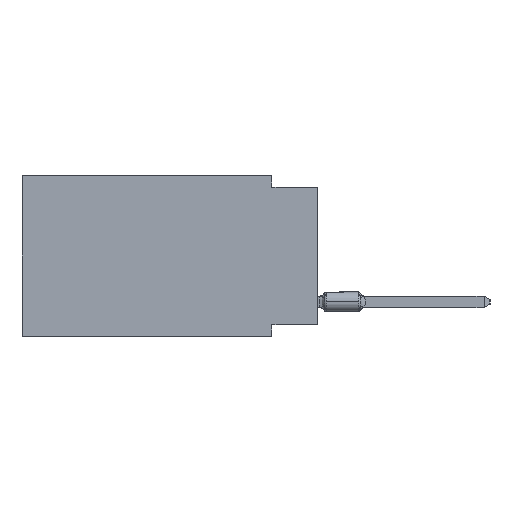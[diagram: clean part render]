
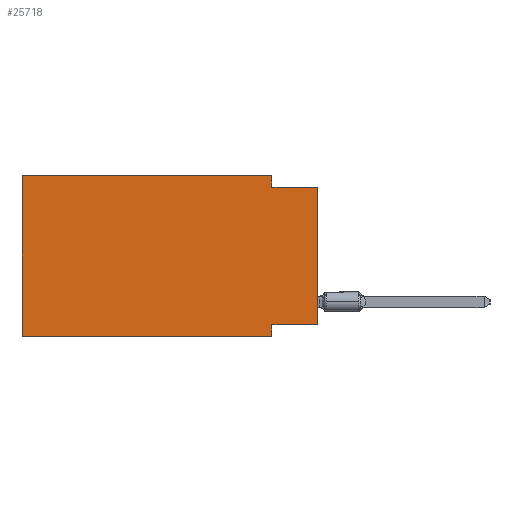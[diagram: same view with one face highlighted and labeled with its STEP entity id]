
A CAD part, left-side view. The second image highlights one B-rep face of the part: STEP entity #25718.
In plain terms, the highlighted planar face has unit normal (-1, 0, 0).
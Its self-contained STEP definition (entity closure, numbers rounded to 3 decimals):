
#2215 = LINE ( 'NONE', #15196, #21872 ) ;
#2265 = DIRECTION ( 'NONE',  ( 0., -1., 0. ) ) ;
#2709 = CARTESIAN_POINT ( 'NONE',  ( 0., 2.54, -8.89 ) ) ;
#3621 = LINE ( 'NONE', #29125, #31498 ) ;
#4980 = CARTESIAN_POINT ( 'NONE',  ( 0., 0., -0.635 ) ) ;
#5808 = EDGE_CURVE ( 'NONE', #7178, #38182, #6358, .T. ) ;
#6358 = LINE ( 'NONE', #35792, #7038 ) ;
#7038 = VECTOR ( 'NONE', #32453, 1000. ) ;
#7178 = VERTEX_POINT ( 'NONE', #31589 ) ;
#7741 = ORIENTED_EDGE ( 'NONE', *, *, #18142, .T. ) ;
#9177 = EDGE_CURVE ( 'NONE', #12048, #35317, #15243, .T. ) ;
#9203 = ORIENTED_EDGE ( 'NONE', *, *, #9177, .F. ) ;
#10192 = CARTESIAN_POINT ( 'NONE',  ( 0., 0., -8.255 ) ) ;
#10745 = DIRECTION ( 'NONE',  ( 0., -1., 0. ) ) ;
#11091 = CARTESIAN_POINT ( 'NONE',  ( 0., 16.383, 0. ) ) ;
#11846 = DIRECTION ( 'NONE',  ( 0., 0., 1. ) ) ;
#12048 = VERTEX_POINT ( 'NONE', #10192 ) ;
#13253 = VECTOR ( 'NONE', #35479, 1000. ) ;
#14845 = VERTEX_POINT ( 'NONE', #4980 ) ;
#15196 = CARTESIAN_POINT ( 'NONE',  ( 0., 0., 0. ) ) ;
#15243 = LINE ( 'NONE', #37995, #39353 ) ;
#15886 = VECTOR ( 'NONE', #40746, 1000. ) ;
#16350 = VERTEX_POINT ( 'NONE', #19687 ) ;
#16980 = PLANE ( 'NONE',  #17020 ) ;
#17020 = AXIS2_PLACEMENT_3D ( 'NONE', #11091, #36781, #39919 ) ;
#17247 = VECTOR ( 'NONE', #2265, 1000. ) ;
#18142 = EDGE_CURVE ( 'NONE', #7178, #28226, #3621, .T. ) ;
#18381 = CARTESIAN_POINT ( 'NONE',  ( 0., 0., -0.635 ) ) ;
#19687 = CARTESIAN_POINT ( 'NONE',  ( 0., 2.54, -0.635 ) ) ;
#19945 = ORIENTED_EDGE ( 'NONE', *, *, #35447, .F. ) ;
#20301 = FACE_OUTER_BOUND ( 'NONE', #33129, .T. ) ;
#20657 = ORIENTED_EDGE ( 'NONE', *, *, #34658, .F. ) ;
#21872 = VECTOR ( 'NONE', #11846, 1000. ) ;
#22324 = DIRECTION ( 'NONE',  ( 0., 1., 0. ) ) ;
#22740 = CARTESIAN_POINT ( 'NONE',  ( 0., 2.54, 0. ) ) ;
#22844 = DIRECTION ( 'NONE',  ( 0., -1., 0. ) ) ;
#25043 = LINE ( 'NONE', #22740, #13253 ) ;
#25348 = EDGE_CURVE ( 'NONE', #38182, #28399, #36027, .T. ) ;
#25436 = ORIENTED_EDGE ( 'NONE', *, *, #5808, .F. ) ;
#25718 = ADVANCED_FACE ( 'NONE', ( #20301 ), #16980, .F. ) ;
#25758 = ORIENTED_EDGE ( 'NONE', *, *, #30278, .T. ) ;
#27751 = ORIENTED_EDGE ( 'NONE', *, *, #25348, .F. ) ;
#27954 = VECTOR ( 'NONE', #10745, 1000. ) ;
#28226 = VERTEX_POINT ( 'NONE', #40559 ) ;
#28399 = VERTEX_POINT ( 'NONE', #38442 ) ;
#29125 = CARTESIAN_POINT ( 'NONE',  ( 0., 16.383, -8.89 ) ) ;
#30278 = EDGE_CURVE ( 'NONE', #12048, #14845, #2215, .T. ) ;
#30291 = CARTESIAN_POINT ( 'NONE',  ( 0., 2.54, -8.255 ) ) ;
#31498 = VECTOR ( 'NONE', #22844, 1000. ) ;
#31589 = CARTESIAN_POINT ( 'NONE',  ( 0., 16.383, -8.89 ) ) ;
#32453 = DIRECTION ( 'NONE',  ( 0., 0., 1. ) ) ;
#33129 = EDGE_LOOP ( 'NONE', ( #25758, #33493, #19945, #27751, #25436, #7741, #20657, #9203 ) ) ;
#33493 = ORIENTED_EDGE ( 'NONE', *, *, #36559, .F. ) ;
#34451 = LINE ( 'NONE', #18381, #17247 ) ;
#34658 = EDGE_CURVE ( 'NONE', #35317, #28226, #40325, .T. ) ;
#35317 = VERTEX_POINT ( 'NONE', #30291 ) ;
#35447 = EDGE_CURVE ( 'NONE', #28399, #16350, #25043, .T. ) ;
#35479 = DIRECTION ( 'NONE',  ( 0., 0., -1. ) ) ;
#35792 = CARTESIAN_POINT ( 'NONE',  ( 0., 16.383, 0. ) ) ;
#36027 = LINE ( 'NONE', #36829, #27954 ) ;
#36559 = EDGE_CURVE ( 'NONE', #16350, #14845, #34451, .T. ) ;
#36781 = DIRECTION ( 'NONE',  ( 1., 0., 0. ) ) ;
#36829 = CARTESIAN_POINT ( 'NONE',  ( 0., 16.383, 0. ) ) ;
#37995 = CARTESIAN_POINT ( 'NONE',  ( 0., 0., -8.255 ) ) ;
#38182 = VERTEX_POINT ( 'NONE', #40059 ) ;
#38442 = CARTESIAN_POINT ( 'NONE',  ( 0., 2.54, 0. ) ) ;
#39353 = VECTOR ( 'NONE', #22324, 1000. ) ;
#39919 = DIRECTION ( 'NONE',  ( 0., 0., -1. ) ) ;
#40059 = CARTESIAN_POINT ( 'NONE',  ( 0., 16.383, 0. ) ) ;
#40325 = LINE ( 'NONE', #2709, #15886 ) ;
#40559 = CARTESIAN_POINT ( 'NONE',  ( 0., 2.54, -8.89 ) ) ;
#40746 = DIRECTION ( 'NONE',  ( 0., 0., -1. ) ) ;
